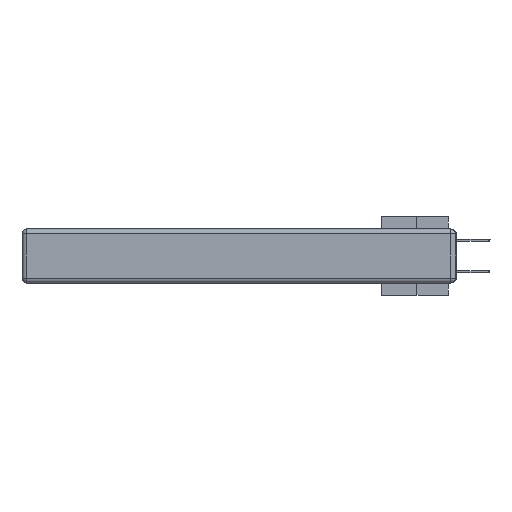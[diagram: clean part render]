
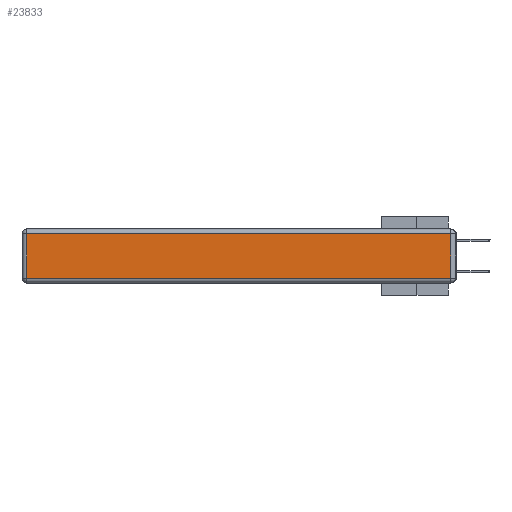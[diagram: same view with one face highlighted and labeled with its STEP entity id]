
A CAD part, left-side view. The second image highlights one B-rep face of the part: STEP entity #23833.
In plain terms, the highlighted planar face has unit normal (-1, 0, 0).
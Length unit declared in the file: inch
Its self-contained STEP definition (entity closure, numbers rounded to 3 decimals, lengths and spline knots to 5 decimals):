
#1148 = CARTESIAN_POINT ( 'NONE',  ( 0., 0., -0.313 ) ) ;
#3444 = LINE ( 'NONE', #1148, #5897 ) ;
#3929 = CARTESIAN_POINT ( 'NONE',  ( 0., 2.72, -0.313 ) ) ;
#4285 = LINE ( 'NONE', #9880, #21908 ) ;
#5092 = LINE ( 'NONE', #11141, #22037 ) ;
#5224 = EDGE_CURVE ( 'NONE', #6792, #30205, #4285, .T. ) ;
#5897 = VECTOR ( 'NONE', #31374, 39.37008 ) ;
#6238 = CARTESIAN_POINT ( 'NONE',  ( 0., 0.03, -0.03 ) ) ;
#6792 = VERTEX_POINT ( 'NONE', #6238 ) ;
#6852 = ORIENTED_EDGE ( 'NONE', *, *, #5224, .T. ) ;
#8489 = ORIENTED_EDGE ( 'NONE', *, *, #15509, .T. ) ;
#9352 = ORIENTED_EDGE ( 'NONE', *, *, #11115, .T. ) ;
#9880 = CARTESIAN_POINT ( 'NONE',  ( 0., 2.75, -0.03 ) ) ;
#9886 = FACE_OUTER_BOUND ( 'NONE', #12290, .T. ) ;
#11115 = EDGE_CURVE ( 'NONE', #28261, #30261, #3444, .T. ) ;
#11141 = CARTESIAN_POINT ( 'NONE',  ( 0., 0.03, -0.343 ) ) ;
#12193 = PLANE ( 'NONE',  #21576 ) ;
#12290 = EDGE_LOOP ( 'NONE', ( #9352, #19745, #6852, #8489 ) ) ;
#12351 = CARTESIAN_POINT ( 'NONE',  ( 0., 0., -0.343 ) ) ;
#13336 = LINE ( 'NONE', #17946, #14381 ) ;
#14381 = VECTOR ( 'NONE', #23377, 39.37008 ) ;
#15509 = EDGE_CURVE ( 'NONE', #30205, #28261, #13336, .T. ) ;
#17946 = CARTESIAN_POINT ( 'NONE',  ( 0., 2.72, -0.343 ) ) ;
#19745 = ORIENTED_EDGE ( 'NONE', *, *, #21357, .T. ) ;
#19934 = DIRECTION ( 'NONE',  ( 0., 1., 0. ) ) ;
#19940 = DIRECTION ( 'NONE',  ( 0., 0., 1. ) ) ;
#20160 = CARTESIAN_POINT ( 'NONE',  ( 0., 0.03, -0.313 ) ) ;
#21357 = EDGE_CURVE ( 'NONE', #30261, #6792, #5092, .T. ) ;
#21576 = AXIS2_PLACEMENT_3D ( 'NONE', #12351, #22394, #19940 ) ;
#21908 = VECTOR ( 'NONE', #19934, 39.37008 ) ;
#22037 = VECTOR ( 'NONE', #26263, 39.37008 ) ;
#22394 = DIRECTION ( 'NONE',  ( -1., 0., 0. ) ) ;
#23377 = DIRECTION ( 'NONE',  ( 0., 0., -1. ) ) ;
#23833 = ADVANCED_FACE ( 'NONE', ( #9886 ), #12193, .T. ) ;
#26263 = DIRECTION ( 'NONE',  ( 0., 0., 1. ) ) ;
#28261 = VERTEX_POINT ( 'NONE', #3929 ) ;
#29180 = CARTESIAN_POINT ( 'NONE',  ( 0., 2.72, -0.03 ) ) ;
#30205 = VERTEX_POINT ( 'NONE', #29180 ) ;
#30261 = VERTEX_POINT ( 'NONE', #20160 ) ;
#31374 = DIRECTION ( 'NONE',  ( 0., -1., 0. ) ) ;
